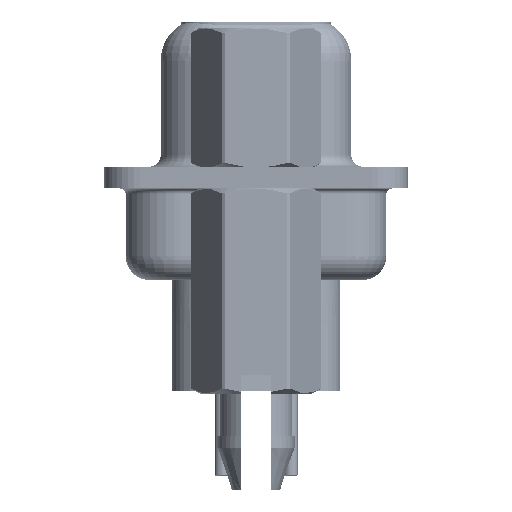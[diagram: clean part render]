
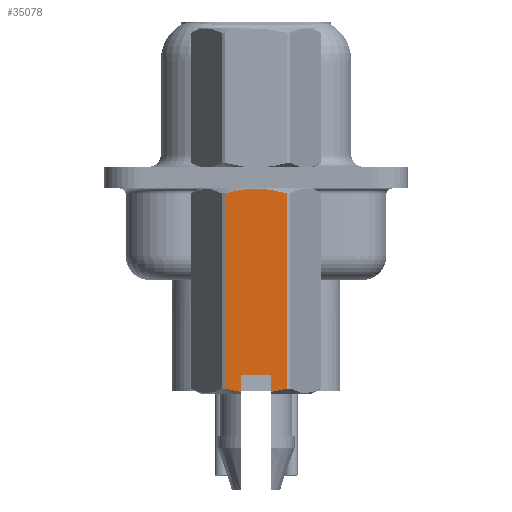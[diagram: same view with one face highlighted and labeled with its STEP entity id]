
A CAD part, left-side view. The second image highlights one B-rep face of the part: STEP entity #35078.
In plain terms, the highlighted planar face has unit normal (-1, 0, 0).
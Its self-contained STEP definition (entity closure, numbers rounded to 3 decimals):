
#224 = ORIENTED_EDGE ( 'NONE', *, *, #50888, .T. ) ;
#349 = EDGE_CURVE ( 'NONE', #26183, #45636, #48564, .T. ) ;
#483 = AXIS2_PLACEMENT_3D ( 'NONE', #14570, #46292, #34589 ) ;
#638 = CARTESIAN_POINT ( 'NONE',  ( -2.381, 0.845, -8.853 ) ) ;
#1560 = CARTESIAN_POINT ( 'NONE',  ( -2.381, 0., -0.468 ) ) ;
#2004 = CARTESIAN_POINT ( 'NONE',  ( -2.381, -0.625, -8.885 ) ) ;
#2228 = VECTOR ( 'NONE', #3555, 1000. ) ;
#2818 = VECTOR ( 'NONE', #37527, 1000. ) ;
#3555 = DIRECTION ( 'NONE',  ( 0., 0., -1. ) ) ;
#5387 = EDGE_CURVE ( 'NONE', #44984, #19691, #18019, .T. ) ;
#5711 = ORIENTED_EDGE ( 'NONE', *, *, #12439, .T. ) ;
#6799 = CARTESIAN_POINT ( 'NONE',  ( -2.381, -0.625, -8.2 ) ) ;
#7379 = CARTESIAN_POINT ( 'NONE',  ( -2.381, -0.842, -8.854 ) ) ;
#7503 = CARTESIAN_POINT ( 'NONE',  ( -2.381, -1.273, 0.581 ) ) ;
#8132 = B_SPLINE_CURVE_WITH_KNOTS ( 'NONE', 3,
 ( #26891, #7379, #16181, #20092 ),
 .UNSPECIFIED., .F., .F.,
 ( 4, 4 ),
 ( 0.003, 0.004 ),
 .UNSPECIFIED. ) ;
#8560 = ORIENTED_EDGE ( 'NONE', *, *, #349, .T. ) ;
#8632 = ORIENTED_EDGE ( 'NONE', *, *, #37570, .T. ) ;
#8857 = LINE ( 'NONE', #24720, #43705 ) ;
#9728 = CARTESIAN_POINT ( 'NONE',  ( -2.381, 1.273, -0.652 ) ) ;
#10665 = ORIENTED_EDGE ( 'NONE', *, *, #37799, .F. ) ;
#11434 = CARTESIAN_POINT ( 'NONE',  ( -2.381, -0.428, -0.485 ) ) ;
#12008 = CARTESIAN_POINT ( 'NONE',  ( -2.381, -1.273, -0.652 ) ) ;
#12439 = EDGE_CURVE ( 'NONE', #42881, #37813, #8132, .T. ) ;
#14570 = CARTESIAN_POINT ( 'NONE',  ( -2.381, -1.375, 7.399 ) ) ;
#14797 = CARTESIAN_POINT ( 'NONE',  ( -2.381, 0.625, -8.885 ) ) ;
#14927 = ORIENTED_EDGE ( 'NONE', *, *, #47593, .T. ) ;
#15327 = CARTESIAN_POINT ( 'NONE',  ( -2.381, -0.853, -0.549 ) ) ;
#15628 = DIRECTION ( 'NONE',  ( 0., 0., -1. ) ) ;
#16181 = CARTESIAN_POINT ( 'NONE',  ( -2.381, -1.06, -8.806 ) ) ;
#16958 = CARTESIAN_POINT ( 'NONE',  ( -2.381, 1.273, -8.748 ) ) ;
#18019 = LINE ( 'NONE', #33366, #2818 ) ;
#18299 = EDGE_CURVE ( 'NONE', #37813, #50398, #23873, .T. ) ;
#18464 = FACE_OUTER_BOUND ( 'NONE', #21094, .T. ) ;
#19026 = CARTESIAN_POINT ( 'NONE',  ( -2.381, -0.625, -8.2 ) ) ;
#19338 = CARTESIAN_POINT ( 'NONE',  ( -2.381, 0.625, -8.2 ) ) ;
#19691 = VERTEX_POINT ( 'NONE', #19338 ) ;
#20092 = CARTESIAN_POINT ( 'NONE',  ( -2.381, -1.273, -8.748 ) ) ;
#20098 = CARTESIAN_POINT ( 'NONE',  ( -2.381, 0.625, -8.885 ) ) ;
#21094 = EDGE_LOOP ( 'NONE', ( #10665, #32704, #8632, #5711, #29719, #21627, #224, #14927, #8560 ) ) ;
#21627 = ORIENTED_EDGE ( 'NONE', *, *, #48982, .T. ) ;
#22899 = CARTESIAN_POINT ( 'NONE',  ( -2.381, -1.065, -0.596 ) ) ;
#23800 = VECTOR ( 'NONE', #15628, 1000. ) ;
#23873 = LINE ( 'NONE', #7503, #43955 ) ;
#24720 = CARTESIAN_POINT ( 'NONE',  ( -2.381, 0.625, -8.2 ) ) ;
#25493 = CARTESIAN_POINT ( 'NONE',  ( -2.381, 1.273, -0.652 ) ) ;
#25847 = CARTESIAN_POINT ( 'NONE',  ( -2.381, 0.858, -0.55 ) ) ;
#26183 = VERTEX_POINT ( 'NONE', #43437 ) ;
#26891 = CARTESIAN_POINT ( 'NONE',  ( -2.381, -0.625, -8.885 ) ) ;
#27065 = CARTESIAN_POINT ( 'NONE',  ( -2.381, -0.215, -0.468 ) ) ;
#29719 = ORIENTED_EDGE ( 'NONE', *, *, #18299, .T. ) ;
#30839 = LINE ( 'NONE', #38890, #2228 ) ;
#30984 = LINE ( 'NONE', #19026, #23800 ) ;
#32603 = CARTESIAN_POINT ( 'NONE',  ( -2.381, 1.066, -0.596 ) ) ;
#32704 = ORIENTED_EDGE ( 'NONE', *, *, #5387, .F. ) ;
#32869 = CARTESIAN_POINT ( 'NONE',  ( -2.381, 0.215, -0.468 ) ) ;
#33366 = CARTESIAN_POINT ( 'NONE',  ( -2.381, -0.625, -8.2 ) ) ;
#34589 = DIRECTION ( 'NONE',  ( 0., 0., 1. ) ) ;
#34990 = VERTEX_POINT ( 'NONE', #1560 ) ;
#35078 = ADVANCED_FACE ( 'NONE', ( #18464 ), #50198, .T. ) ;
#35957 = CARTESIAN_POINT ( 'NONE',  ( -2.381, 1.06, -8.806 ) ) ;
#36664 = DIRECTION ( 'NONE',  ( 0., 0., -1. ) ) ;
#37433 = B_SPLINE_CURVE_WITH_KNOTS ( 'NONE', 3,
 ( #45590, #32869, #48744, #25847, #32603, #9728 ),
 .UNSPECIFIED., .F., .F.,
 ( 4, 2, 4 ),
 ( 0.004, 0.004, 0.005 ),
 .UNSPECIFIED. ) ;
#37527 = DIRECTION ( 'NONE',  ( 0., 1., 0. ) ) ;
#37570 = EDGE_CURVE ( 'NONE', #44984, #42881, #30984, .T. ) ;
#37799 = EDGE_CURVE ( 'NONE', #19691, #45636, #8857, .T. ) ;
#37813 = VERTEX_POINT ( 'NONE', #43693 ) ;
#38890 = CARTESIAN_POINT ( 'NONE',  ( -2.381, 1.273, 0.581 ) ) ;
#39404 = VERTEX_POINT ( 'NONE', #25493 ) ;
#39711 = DIRECTION ( 'NONE',  ( 0., 0., 1. ) ) ;
#42881 = VERTEX_POINT ( 'NONE', #2004 ) ;
#43084 = B_SPLINE_CURVE_WITH_KNOTS ( 'NONE', 3,
 ( #46285, #22899, #15327, #11434, #27065, #51218 ),
 .UNSPECIFIED., .F., .F.,
 ( 4, 2, 4 ),
 ( 0.003, 0.003, 0.004 ),
 .UNSPECIFIED. ) ;
#43437 = CARTESIAN_POINT ( 'NONE',  ( -2.381, 1.273, -8.748 ) ) ;
#43693 = CARTESIAN_POINT ( 'NONE',  ( -2.381, -1.273, -8.748 ) ) ;
#43705 = VECTOR ( 'NONE', #36664, 1000. ) ;
#43955 = VECTOR ( 'NONE', #39711, 1000. ) ;
#44984 = VERTEX_POINT ( 'NONE', #6799 ) ;
#45590 = CARTESIAN_POINT ( 'NONE',  ( -2.381, 0., -0.468 ) ) ;
#45636 = VERTEX_POINT ( 'NONE', #14797 ) ;
#46285 = CARTESIAN_POINT ( 'NONE',  ( -2.381, -1.273, -0.652 ) ) ;
#46292 = DIRECTION ( 'NONE',  ( -1., 0., 0. ) ) ;
#47593 = EDGE_CURVE ( 'NONE', #39404, #26183, #30839, .T. ) ;
#48564 = B_SPLINE_CURVE_WITH_KNOTS ( 'NONE', 3,
 ( #16958, #35957, #638, #20098 ),
 .UNSPECIFIED., .F., .F.,
 ( 4, 4 ),
 ( 0.001, 0.002 ),
 .UNSPECIFIED. ) ;
#48744 = CARTESIAN_POINT ( 'NONE',  ( -2.381, 0.432, -0.485 ) ) ;
#48982 = EDGE_CURVE ( 'NONE', #50398, #34990, #43084, .T. ) ;
#50198 = PLANE ( 'NONE',  #483 ) ;
#50398 = VERTEX_POINT ( 'NONE', #12008 ) ;
#50888 = EDGE_CURVE ( 'NONE', #34990, #39404, #37433, .T. ) ;
#51218 = CARTESIAN_POINT ( 'NONE',  ( -2.381, 0., -0.468 ) ) ;
